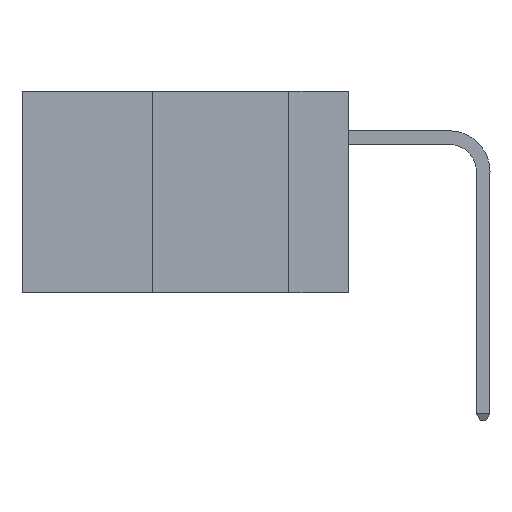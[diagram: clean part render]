
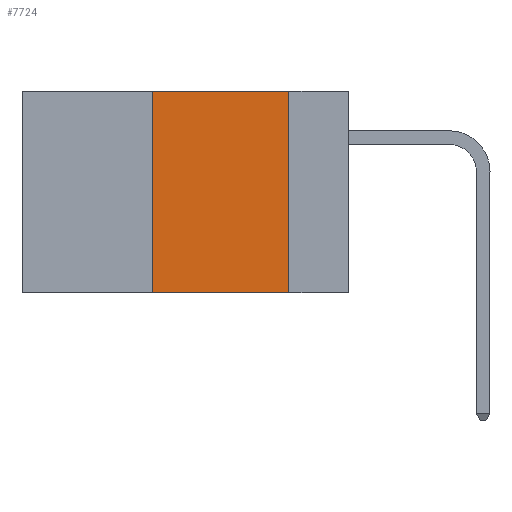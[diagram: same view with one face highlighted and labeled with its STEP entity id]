
A CAD part, left-side view. The second image highlights one B-rep face of the part: STEP entity #7724.
In plain terms, the highlighted planar face has unit normal (-1, 0, 0).
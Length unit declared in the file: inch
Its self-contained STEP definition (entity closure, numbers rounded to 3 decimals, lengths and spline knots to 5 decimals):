
#42 = LINE ( 'NONE', #7246, #7369 ) ;
#1276 = DIRECTION ( 'NONE',  ( 0., 0., -1. ) ) ;
#1381 = VERTEX_POINT ( 'NONE', #6315 ) ;
#4061 = ORIENTED_EDGE ( 'NONE', *, *, #6581, .F. ) ;
#4195 = FACE_OUTER_BOUND ( 'NONE', #8064, .T. ) ;
#4724 = DIRECTION ( 'NONE',  ( 1., 0., 0. ) ) ;
#5093 = CARTESIAN_POINT ( 'NONE',  ( 0., 0.36, 0. ) ) ;
#5176 = CARTESIAN_POINT ( 'NONE',  ( 0., 0.6, 0. ) ) ;
#6315 = CARTESIAN_POINT ( 'NONE',  ( 0., 0.11, 0. ) ) ;
#6581 = EDGE_CURVE ( 'NONE', #15694, #17127, #15889, .T. ) ;
#7246 = CARTESIAN_POINT ( 'NONE',  ( 0., 0.6, -0.37 ) ) ;
#7369 = VECTOR ( 'NONE', #8665, 39.37008 ) ;
#7724 = ADVANCED_FACE ( 'NONE', ( #4195 ), #10367, .F. ) ;
#7847 = CARTESIAN_POINT ( 'NONE',  ( 0., 0.36, 0. ) ) ;
#8064 = EDGE_LOOP ( 'NONE', ( #15168, #14072, #4061, #8849 ) ) ;
#8665 = DIRECTION ( 'NONE',  ( 0., -1., 0. ) ) ;
#8709 = VECTOR ( 'NONE', #1276, 39.37008 ) ;
#8849 = ORIENTED_EDGE ( 'NONE', *, *, #16830, .T. ) ;
#9196 = CARTESIAN_POINT ( 'NONE',  ( 0., 0.11, -0.37 ) ) ;
#9661 = EDGE_CURVE ( 'NONE', #17127, #1381, #11884, .T. ) ;
#10367 = PLANE ( 'NONE',  #13065 ) ;
#10954 = EDGE_CURVE ( 'NONE', #1381, #15901, #12443, .T. ) ;
#11884 = LINE ( 'NONE', #5176, #15187 ) ;
#12236 = VECTOR ( 'NONE', #16163, 39.37008 ) ;
#12443 = LINE ( 'NONE', #16770, #8709 ) ;
#12893 = CARTESIAN_POINT ( 'NONE',  ( 0., 0.36, -0.37 ) ) ;
#13065 = AXIS2_PLACEMENT_3D ( 'NONE', #13253, #4724, #14611 ) ;
#13253 = CARTESIAN_POINT ( 'NONE',  ( 0., 0.6, 0. ) ) ;
#14072 = ORIENTED_EDGE ( 'NONE', *, *, #9661, .F. ) ;
#14611 = DIRECTION ( 'NONE',  ( 0., 0., -1. ) ) ;
#15033 = DIRECTION ( 'NONE',  ( 0., -1., 0. ) ) ;
#15168 = ORIENTED_EDGE ( 'NONE', *, *, #10954, .F. ) ;
#15187 = VECTOR ( 'NONE', #15033, 39.37008 ) ;
#15694 = VERTEX_POINT ( 'NONE', #12893 ) ;
#15889 = LINE ( 'NONE', #7847, #12236 ) ;
#15901 = VERTEX_POINT ( 'NONE', #9196 ) ;
#16163 = DIRECTION ( 'NONE',  ( 0., 0., 1. ) ) ;
#16770 = CARTESIAN_POINT ( 'NONE',  ( 0., 0.11, 0. ) ) ;
#16830 = EDGE_CURVE ( 'NONE', #15694, #15901, #42, .T. ) ;
#17127 = VERTEX_POINT ( 'NONE', #5093 ) ;
